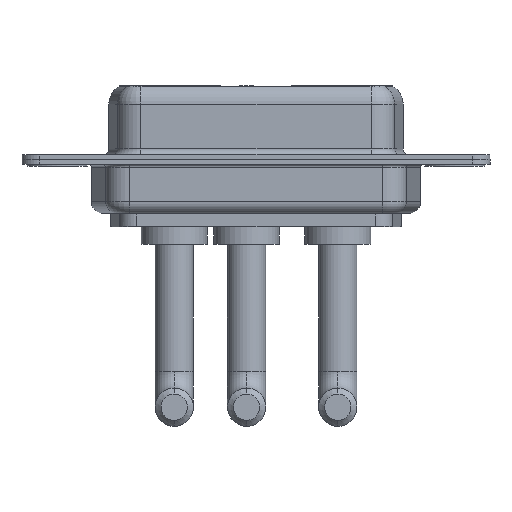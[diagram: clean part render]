
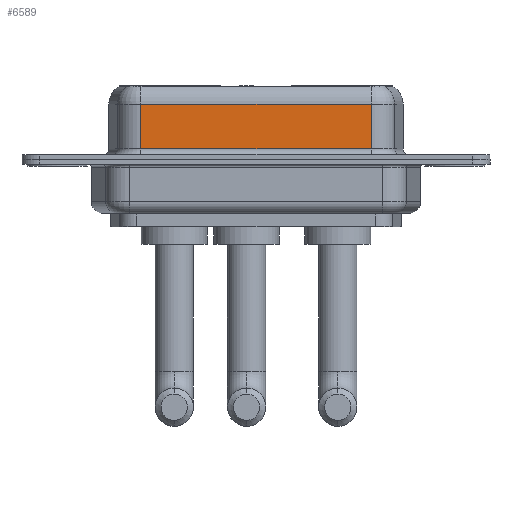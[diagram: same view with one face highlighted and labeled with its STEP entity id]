
A CAD part, front view. The second image highlights one B-rep face of the part: STEP entity #6589.
In plain terms, the highlighted planar face has unit normal (0, -1, 0).
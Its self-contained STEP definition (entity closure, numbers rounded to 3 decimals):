
#583 = ORIENTED_EDGE ( 'NONE', *, *, #9064, .T. ) ;
#982 = CARTESIAN_POINT ( 'NONE',  ( 7.013, -3.95, 4.65 ) ) ;
#1567 = CARTESIAN_POINT ( 'NONE',  ( 26.287, -3.95, 6.4 ) ) ;
#1728 = VECTOR ( 'NONE', #9130, 1000. ) ;
#1891 = DIRECTION ( 'NONE',  ( 0., 0., -1. ) ) ;
#2105 = DIRECTION ( 'NONE',  ( 0., 1., 0. ) ) ;
#2146 = CARTESIAN_POINT ( 'NONE',  ( 26.287, -3.95, 4.65 ) ) ;
#2254 = VECTOR ( 'NONE', #2572, 1000. ) ;
#2572 = DIRECTION ( 'NONE',  ( 0., 0., -1. ) ) ;
#2832 = CARTESIAN_POINT ( 'NONE',  ( 26.287, -3.95, 6.4 ) ) ;
#3859 = FACE_OUTER_BOUND ( 'NONE', #7805, .T. ) ;
#4197 = DIRECTION ( 'NONE',  ( -1., 0., 0. ) ) ;
#5288 = LINE ( 'NONE', #8895, #1728 ) ;
#5311 = LINE ( 'NONE', #1567, #2254 ) ;
#6032 = LINE ( 'NONE', #2146, #8291 ) ;
#6333 = AXIS2_PLACEMENT_3D ( 'NONE', #2832, #2105, #9333 ) ;
#6391 = LINE ( 'NONE', #9794, #9586 ) ;
#6398 = VERTEX_POINT ( 'NONE', #11597 ) ;
#6515 = ORIENTED_EDGE ( 'NONE', *, *, #11698, .T. ) ;
#6589 = ADVANCED_FACE ( 'NONE', ( #3859 ), #7460, .F. ) ;
#6867 = EDGE_CURVE ( 'NONE', #7202, #8266, #5311, .T. ) ;
#7194 = EDGE_CURVE ( 'NONE', #7202, #7830, #6032, .T. ) ;
#7202 = VERTEX_POINT ( 'NONE', #7804 ) ;
#7203 = CARTESIAN_POINT ( 'NONE',  ( 26.287, -3.95, 0.9 ) ) ;
#7460 = PLANE ( 'NONE',  #6333 ) ;
#7749 = ORIENTED_EDGE ( 'NONE', *, *, #7194, .T. ) ;
#7804 = CARTESIAN_POINT ( 'NONE',  ( 26.287, -3.95, 4.65 ) ) ;
#7805 = EDGE_LOOP ( 'NONE', ( #11815, #7749, #6515, #583 ) ) ;
#7830 = VERTEX_POINT ( 'NONE', #982 ) ;
#8266 = VERTEX_POINT ( 'NONE', #7203 ) ;
#8291 = VECTOR ( 'NONE', #4197, 1000. ) ;
#8895 = CARTESIAN_POINT ( 'NONE',  ( 26.287, -3.95, 0.9 ) ) ;
#9064 = EDGE_CURVE ( 'NONE', #6398, #8266, #5288, .T. ) ;
#9130 = DIRECTION ( 'NONE',  ( 1., 0., 0. ) ) ;
#9333 = DIRECTION ( 'NONE',  ( 0., 0., 1. ) ) ;
#9586 = VECTOR ( 'NONE', #1891, 1000. ) ;
#9794 = CARTESIAN_POINT ( 'NONE',  ( 7.013, -3.95, 6.4 ) ) ;
#11597 = CARTESIAN_POINT ( 'NONE',  ( 7.013, -3.95, 0.9 ) ) ;
#11698 = EDGE_CURVE ( 'NONE', #7830, #6398, #6391, .T. ) ;
#11815 = ORIENTED_EDGE ( 'NONE', *, *, #6867, .F. ) ;
